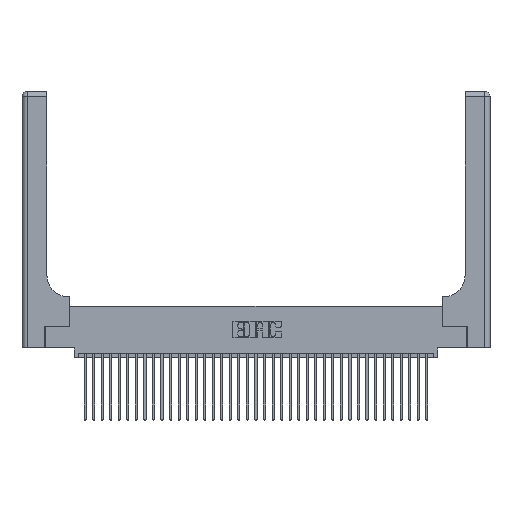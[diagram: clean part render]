
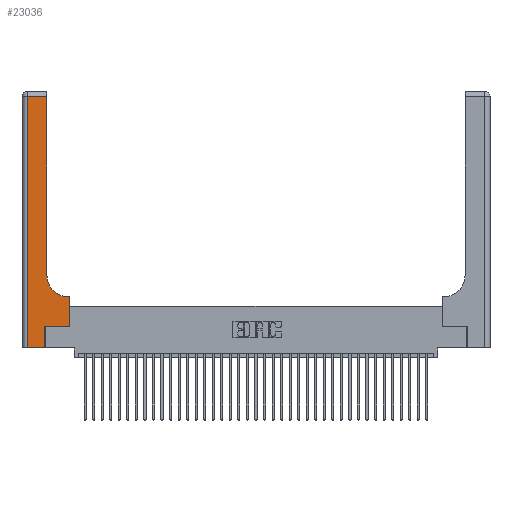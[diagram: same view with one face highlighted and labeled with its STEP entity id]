
A CAD part, top view. The second image highlights one B-rep face of the part: STEP entity #23036.
In plain terms, the highlighted planar face has unit normal (0, 0, 1).
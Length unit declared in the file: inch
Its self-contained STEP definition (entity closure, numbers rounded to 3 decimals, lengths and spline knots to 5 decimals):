
#539 = AXIS2_PLACEMENT_3D ( 'NONE', #5213, #19335, #1443 ) ;
#808 = CARTESIAN_POINT ( 'NONE',  ( 0.269, 0.25, 0.37 ) ) ;
#1296 = DIRECTION ( 'NONE',  ( -1., 0., 0. ) ) ;
#1443 = DIRECTION ( 'NONE',  ( 1., 0., 0. ) ) ;
#2137 = VERTEX_POINT ( 'NONE', #31719 ) ;
#3562 = VECTOR ( 'NONE', #12834, 39.37008 ) ;
#3654 = LINE ( 'NONE', #17540, #31851 ) ;
#3990 = EDGE_CURVE ( 'NONE', #13040, #8990, #24456, .T. ) ;
#4278 = CARTESIAN_POINT ( 'NONE',  ( 0., 2.94, 0.37 ) ) ;
#4341 = EDGE_CURVE ( 'NONE', #19928, #2137, #22805, .T. ) ;
#4399 = EDGE_CURVE ( 'NONE', #2137, #18958, #8620, .T. ) ;
#4483 = DIRECTION ( 'NONE',  ( 0., 0., -1. ) ) ;
#5000 = VERTEX_POINT ( 'NONE', #808 ) ;
#5213 = CARTESIAN_POINT ( 'NONE',  ( 0.5415, 0.85, 0.37 ) ) ;
#6915 = VECTOR ( 'NONE', #20843, 39.37008 ) ;
#8078 = DIRECTION ( 'NONE',  ( 0., 1., 0. ) ) ;
#8136 = VERTEX_POINT ( 'NONE', #14774 ) ;
#8376 = CARTESIAN_POINT ( 'NONE',  ( 0.5585, 0.25, 0.37 ) ) ;
#8620 = LINE ( 'NONE', #4278, #3562 ) ;
#8990 = VERTEX_POINT ( 'NONE', #30492 ) ;
#10906 = ORIENTED_EDGE ( 'NONE', *, *, #27312, .T. ) ;
#11282 = CARTESIAN_POINT ( 'NONE',  ( 0.2915, 3., 0.37 ) ) ;
#11540 = ORIENTED_EDGE ( 'NONE', *, *, #4399, .T. ) ;
#12456 = CARTESIAN_POINT ( 'NONE',  ( 0.06, 2.94, 0.37 ) ) ;
#12697 = VECTOR ( 'NONE', #20196, 39.37008 ) ;
#12834 = DIRECTION ( 'NONE',  ( -1., 0., 0. ) ) ;
#12977 = DIRECTION ( 'NONE',  ( 1., 0., 0. ) ) ;
#13040 = VERTEX_POINT ( 'NONE', #21363 ) ;
#13891 = VECTOR ( 'NONE', #21032, 39.37008 ) ;
#14114 = EDGE_CURVE ( 'NONE', #8136, #5000, #24198, .T. ) ;
#14222 = VECTOR ( 'NONE', #12977, 39.37008 ) ;
#14231 = DIRECTION ( 'NONE',  ( -1., 0., 0. ) ) ;
#14238 = DIRECTION ( 'NONE',  ( 0., -1., 0. ) ) ;
#14774 = CARTESIAN_POINT ( 'NONE',  ( 0.269, 0., 0.37 ) ) ;
#14827 = VERTEX_POINT ( 'NONE', #36836 ) ;
#15040 = CARTESIAN_POINT ( 'NONE',  ( 0.2915, 0.85, 0.37 ) ) ;
#17408 = LINE ( 'NONE', #33658, #14222 ) ;
#17415 = ORIENTED_EDGE ( 'NONE', *, *, #4341, .T. ) ;
#17540 = CARTESIAN_POINT ( 'NONE',  ( 0.2915, 0.6, 0.37 ) ) ;
#17867 = EDGE_CURVE ( 'NONE', #18958, #33731, #27887, .T. ) ;
#17947 = FACE_OUTER_BOUND ( 'NONE', #27131, .T. ) ;
#18753 = PLANE ( 'NONE',  #35494 ) ;
#18958 = VERTEX_POINT ( 'NONE', #12456 ) ;
#19335 = DIRECTION ( 'NONE',  ( 0., 0., -1. ) ) ;
#19360 = ORIENTED_EDGE ( 'NONE', *, *, #36816, .T. ) ;
#19503 = CIRCLE ( 'NONE', #539, 0.25 ) ;
#19743 = EDGE_CURVE ( 'NONE', #14827, #19928, #19503, .T. ) ;
#19928 = VERTEX_POINT ( 'NONE', #15040 ) ;
#20196 = DIRECTION ( 'NONE',  ( 0., 1., 0. ) ) ;
#20843 = DIRECTION ( 'NONE',  ( 0., 1., 0. ) ) ;
#21032 = DIRECTION ( 'NONE',  ( 1., 0., 0. ) ) ;
#21363 = CARTESIAN_POINT ( 'NONE',  ( 0.5585, 0.25, 0.37 ) ) ;
#21518 = ORIENTED_EDGE ( 'NONE', *, *, #19743, .T. ) ;
#22805 = LINE ( 'NONE', #11282, #35566 ) ;
#23036 = ADVANCED_FACE ( 'NONE', ( #17947 ), #18753, .F. ) ;
#23558 = CARTESIAN_POINT ( 'NONE',  ( 0., 0., 0.37 ) ) ;
#24198 = LINE ( 'NONE', #35362, #6915 ) ;
#24456 = LINE ( 'NONE', #8376, #12697 ) ;
#25104 = ORIENTED_EDGE ( 'NONE', *, *, #14114, .T. ) ;
#25113 = VECTOR ( 'NONE', #14238, 39.37008 ) ;
#27131 = EDGE_LOOP ( 'NONE', ( #17415, #11540, #33000, #27241, #25104, #19360, #30617, #10906, #21518 ) ) ;
#27241 = ORIENTED_EDGE ( 'NONE', *, *, #35259, .T. ) ;
#27312 = EDGE_CURVE ( 'NONE', #8990, #14827, #3654, .T. ) ;
#27712 = CARTESIAN_POINT ( 'NONE',  ( 0.06, 0., 0.37 ) ) ;
#27887 = LINE ( 'NONE', #31518, #25113 ) ;
#30492 = CARTESIAN_POINT ( 'NONE',  ( 0.5585, 0.6, 0.37 ) ) ;
#30617 = ORIENTED_EDGE ( 'NONE', *, *, #3990, .T. ) ;
#31518 = CARTESIAN_POINT ( 'NONE',  ( 0.06, 3., 0.37 ) ) ;
#31719 = CARTESIAN_POINT ( 'NONE',  ( 0.2915, 2.94, 0.37 ) ) ;
#31851 = VECTOR ( 'NONE', #14231, 39.37008 ) ;
#32108 = LINE ( 'NONE', #23558, #13891 ) ;
#33000 = ORIENTED_EDGE ( 'NONE', *, *, #17867, .T. ) ;
#33658 = CARTESIAN_POINT ( 'NONE',  ( 0.269, 0.25, 0.37 ) ) ;
#33731 = VERTEX_POINT ( 'NONE', #27712 ) ;
#35259 = EDGE_CURVE ( 'NONE', #33731, #8136, #32108, .T. ) ;
#35362 = CARTESIAN_POINT ( 'NONE',  ( 0.269, 0., 0.37 ) ) ;
#35494 = AXIS2_PLACEMENT_3D ( 'NONE', #36150, #4483, #1296 ) ;
#35566 = VECTOR ( 'NONE', #8078, 39.37008 ) ;
#36150 = CARTESIAN_POINT ( 'NONE',  ( 0., 3., 0.37 ) ) ;
#36816 = EDGE_CURVE ( 'NONE', #5000, #13040, #17408, .T. ) ;
#36836 = CARTESIAN_POINT ( 'NONE',  ( 0.5415, 0.6, 0.37 ) ) ;
